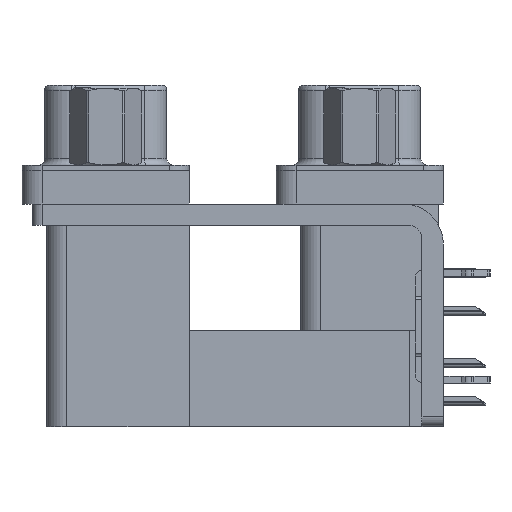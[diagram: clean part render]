
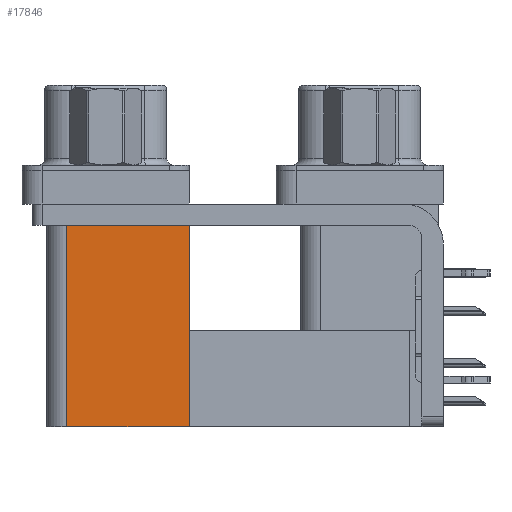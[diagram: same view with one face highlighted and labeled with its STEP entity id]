
A CAD part, left-side view. The second image highlights one B-rep face of the part: STEP entity #17846.
In plain terms, the highlighted planar face has unit normal (-1, 0, 0).
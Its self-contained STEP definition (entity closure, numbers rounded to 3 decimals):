
#46 = VECTOR ( 'NONE', #5957, 1000. ) ;
#3722 = PLANE ( 'NONE',  #23328 ) ;
#4311 = LINE ( 'NONE', #19299, #17079 ) ;
#4768 = VERTEX_POINT ( 'NONE', #44899 ) ;
#5547 = DIRECTION ( 'NONE',  ( 0., 0., 1. ) ) ;
#5957 = DIRECTION ( 'NONE',  ( 0., 1., 0. ) ) ;
#8147 = CARTESIAN_POINT ( 'NONE',  ( 3.7, 12.775, -2.5 ) ) ;
#8354 = VECTOR ( 'NONE', #5547, 1000. ) ;
#9480 = CARTESIAN_POINT ( 'NONE',  ( 3.7, 21.975, -2.5 ) ) ;
#10730 = DIRECTION ( 'NONE',  ( 1., 0., 0. ) ) ;
#11440 = FACE_OUTER_BOUND ( 'NONE', #19082, .T. ) ;
#13222 = CARTESIAN_POINT ( 'NONE',  ( 3.7, 12.775, -19.2 ) ) ;
#14283 = EDGE_CURVE ( 'NONE', #37442, #4768, #46335, .T. ) ;
#14372 = DIRECTION ( 'NONE',  ( 0., 1., 0. ) ) ;
#16503 = EDGE_CURVE ( 'NONE', #38461, #36116, #4311, .T. ) ;
#17059 = ORIENTED_EDGE ( 'NONE', *, *, #19896, .F. ) ;
#17079 = VECTOR ( 'NONE', #30409, 1000. ) ;
#17846 = ADVANCED_FACE ( 'NONE', ( #11440 ), #3722, .F. ) ;
#18139 = CARTESIAN_POINT ( 'NONE',  ( 3.7, 21.975, -19.2 ) ) ;
#19082 = EDGE_LOOP ( 'NONE', ( #31097, #17059, #35989, #47757 ) ) ;
#19299 = CARTESIAN_POINT ( 'NONE',  ( 3.7, 12.775, -2.5 ) ) ;
#19633 = VECTOR ( 'NONE', #43997, 1000. ) ;
#19896 = EDGE_CURVE ( 'NONE', #4768, #36116, #39884, .T. ) ;
#23328 = AXIS2_PLACEMENT_3D ( 'NONE', #32750, #10730, #14372 ) ;
#23778 = CARTESIAN_POINT ( 'NONE',  ( 3.7, 12.775, -19.2 ) ) ;
#30409 = DIRECTION ( 'NONE',  ( 0., 1., 0. ) ) ;
#31097 = ORIENTED_EDGE ( 'NONE', *, *, #16503, .T. ) ;
#32750 = CARTESIAN_POINT ( 'NONE',  ( 3.7, 12.775, -19.2 ) ) ;
#34578 = CARTESIAN_POINT ( 'NONE',  ( 3.7, 12.775, -19.2 ) ) ;
#35146 = EDGE_CURVE ( 'NONE', #37442, #38461, #45214, .T. ) ;
#35989 = ORIENTED_EDGE ( 'NONE', *, *, #14283, .F. ) ;
#36116 = VERTEX_POINT ( 'NONE', #9480 ) ;
#37442 = VERTEX_POINT ( 'NONE', #23778 ) ;
#38461 = VERTEX_POINT ( 'NONE', #8147 ) ;
#39884 = LINE ( 'NONE', #18139, #19633 ) ;
#43997 = DIRECTION ( 'NONE',  ( 0., 0., 1. ) ) ;
#44899 = CARTESIAN_POINT ( 'NONE',  ( 3.7, 21.975, -19.2 ) ) ;
#45214 = LINE ( 'NONE', #34578, #8354 ) ;
#46335 = LINE ( 'NONE', #13222, #46 ) ;
#47757 = ORIENTED_EDGE ( 'NONE', *, *, #35146, .T. ) ;
